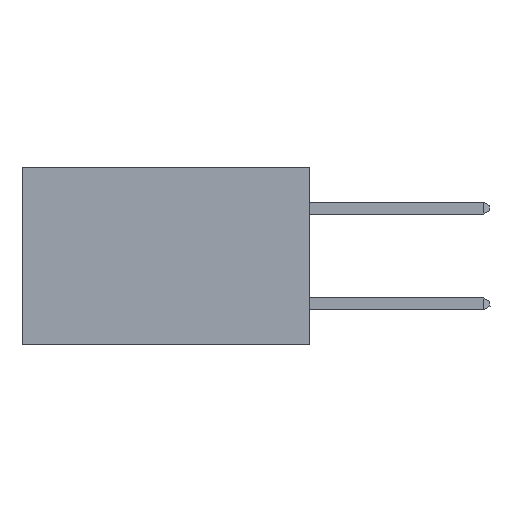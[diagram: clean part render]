
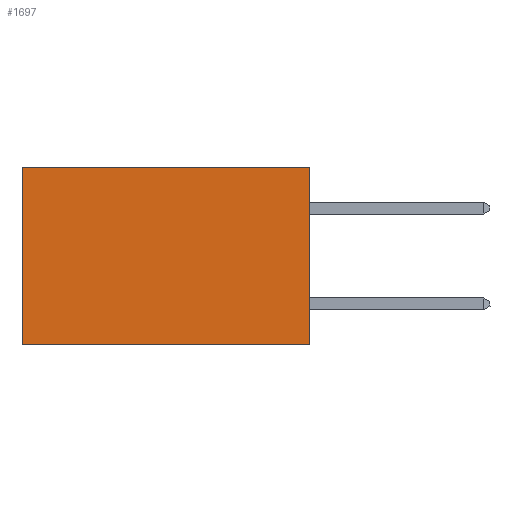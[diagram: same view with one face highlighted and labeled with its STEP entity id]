
A CAD part, left-side view. The second image highlights one B-rep face of the part: STEP entity #1697.
In plain terms, the highlighted planar face has unit normal (-1, 0, 0).
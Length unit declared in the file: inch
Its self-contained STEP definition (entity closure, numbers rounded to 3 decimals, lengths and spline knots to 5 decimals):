
#385 = VECTOR ( 'NONE', #2809, 39.37008 ) ;
#572 = EDGE_CURVE ( 'NONE', #9617, #4298, #9618, .T. ) ;
#822 = ORIENTED_EDGE ( 'NONE', *, *, #13465, .T. ) ;
#1697 = ADVANCED_FACE ( 'NONE', ( #11458 ), #9585, .F. ) ;
#1989 = VECTOR ( 'NONE', #10616, 39.37008 ) ;
#2196 = CARTESIAN_POINT ( 'NONE',  ( 0.2875, 0.6, -0.37 ) ) ;
#2584 = VERTEX_POINT ( 'NONE', #4770 ) ;
#2732 = DIRECTION ( 'NONE',  ( 1., 0., 0. ) ) ;
#2809 = DIRECTION ( 'NONE',  ( 0., 1., 0. ) ) ;
#3368 = CARTESIAN_POINT ( 'NONE',  ( 0.2875, 0., 0. ) ) ;
#3410 = ORIENTED_EDGE ( 'NONE', *, *, #6545, .F. ) ;
#3903 = CARTESIAN_POINT ( 'NONE',  ( 0.2875, 0., 0. ) ) ;
#4298 = VERTEX_POINT ( 'NONE', #2196 ) ;
#4770 = CARTESIAN_POINT ( 'NONE',  ( 0.2875, 0.6, 0. ) ) ;
#4907 = DIRECTION ( 'NONE',  ( 0., 0., -1. ) ) ;
#5511 = VECTOR ( 'NONE', #12305, 39.37008 ) ;
#5543 = ORIENTED_EDGE ( 'NONE', *, *, #13209, .T. ) ;
#5825 = LINE ( 'NONE', #3368, #1989 ) ;
#6384 = CARTESIAN_POINT ( 'NONE',  ( 0.2875, 0., -0.37 ) ) ;
#6545 = EDGE_CURVE ( 'NONE', #11334, #9617, #5825, .T. ) ;
#7161 = LINE ( 'NONE', #8450, #8941 ) ;
#7605 = CARTESIAN_POINT ( 'NONE',  ( 0.2875, 0., 0. ) ) ;
#8450 = CARTESIAN_POINT ( 'NONE',  ( 0.2875, 0.6, 0. ) ) ;
#8941 = VECTOR ( 'NONE', #4907, 39.37008 ) ;
#9585 = PLANE ( 'NONE',  #11529 ) ;
#9617 = VERTEX_POINT ( 'NONE', #14273 ) ;
#9618 = LINE ( 'NONE', #6384, #385 ) ;
#10150 = EDGE_LOOP ( 'NONE', ( #5543, #11012, #3410, #822 ) ) ;
#10616 = DIRECTION ( 'NONE',  ( 0., 0., -1. ) ) ;
#10792 = DIRECTION ( 'NONE',  ( 0., 0., -1. ) ) ;
#11012 = ORIENTED_EDGE ( 'NONE', *, *, #572, .F. ) ;
#11334 = VERTEX_POINT ( 'NONE', #12216 ) ;
#11458 = FACE_OUTER_BOUND ( 'NONE', #10150, .T. ) ;
#11529 = AXIS2_PLACEMENT_3D ( 'NONE', #3903, #2732, #10792 ) ;
#12216 = CARTESIAN_POINT ( 'NONE',  ( 0.2875, 0., 0. ) ) ;
#12250 = LINE ( 'NONE', #7605, #5511 ) ;
#12305 = DIRECTION ( 'NONE',  ( 0., 1., 0. ) ) ;
#13209 = EDGE_CURVE ( 'NONE', #2584, #4298, #7161, .T. ) ;
#13465 = EDGE_CURVE ( 'NONE', #11334, #2584, #12250, .T. ) ;
#14273 = CARTESIAN_POINT ( 'NONE',  ( 0.2875, 0., -0.37 ) ) ;
